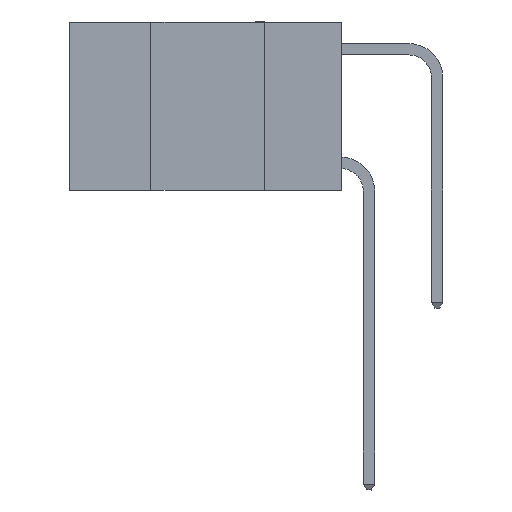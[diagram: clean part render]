
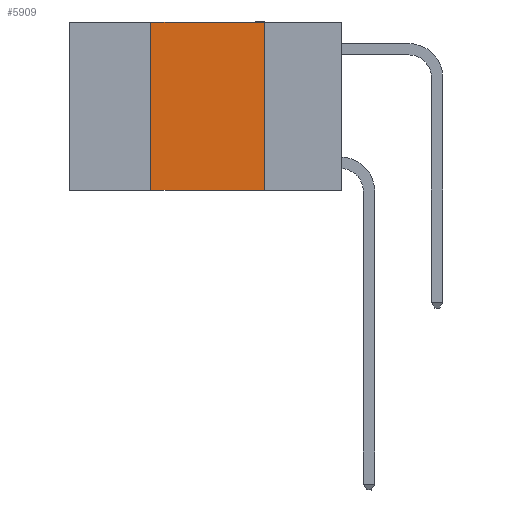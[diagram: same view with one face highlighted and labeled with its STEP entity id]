
A CAD part, left-side view. The second image highlights one B-rep face of the part: STEP entity #5909.
In plain terms, the highlighted planar face has unit normal (-1, 0, 0).
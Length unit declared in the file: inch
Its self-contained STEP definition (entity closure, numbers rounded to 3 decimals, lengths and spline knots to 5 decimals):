
#343 = VERTEX_POINT ( 'NONE', #6708 ) ;
#415 = VECTOR ( 'NONE', #12996, 39.37008 ) ;
#549 = CARTESIAN_POINT ( 'NONE',  ( 0., 0.17, 0. ) ) ;
#1062 = ORIENTED_EDGE ( 'NONE', *, *, #9405, .F. ) ;
#1508 = AXIS2_PLACEMENT_3D ( 'NONE', #9633, #1908, #12872 ) ;
#1541 = ORIENTED_EDGE ( 'NONE', *, *, #9447, .F. ) ;
#1908 = DIRECTION ( 'NONE',  ( 1., 0., 0. ) ) ;
#2090 = FACE_OUTER_BOUND ( 'NONE', #12946, .T. ) ;
#2152 = DIRECTION ( 'NONE',  ( 0., 0., 1. ) ) ;
#2415 = VECTOR ( 'NONE', #8835, 39.37008 ) ;
#2990 = VERTEX_POINT ( 'NONE', #5222 ) ;
#5222 = CARTESIAN_POINT ( 'NONE',  ( 0., 0.42, -0.37 ) ) ;
#5909 = ADVANCED_FACE ( 'NONE', ( #2090 ), #18929, .F. ) ;
#6468 = LINE ( 'NONE', #7260, #2415 ) ;
#6708 = CARTESIAN_POINT ( 'NONE',  ( 0., 0.17, 0. ) ) ;
#7260 = CARTESIAN_POINT ( 'NONE',  ( 0., 0.6, 0. ) ) ;
#7269 = CARTESIAN_POINT ( 'NONE',  ( 0., 0.17, -0.37 ) ) ;
#8835 = DIRECTION ( 'NONE',  ( 0., -1., 0. ) ) ;
#9405 = EDGE_CURVE ( 'NONE', #343, #10947, #12389, .T. ) ;
#9447 = EDGE_CURVE ( 'NONE', #2990, #9771, #11911, .T. ) ;
#9500 = EDGE_CURVE ( 'NONE', #2990, #10947, #18613, .T. ) ;
#9633 = CARTESIAN_POINT ( 'NONE',  ( 0., 0.6, 0. ) ) ;
#9771 = VERTEX_POINT ( 'NONE', #17113 ) ;
#9808 = ORIENTED_EDGE ( 'NONE', *, *, #9500, .T. ) ;
#10111 = DIRECTION ( 'NONE',  ( 0., -1., 0. ) ) ;
#10947 = VERTEX_POINT ( 'NONE', #7269 ) ;
#11392 = VECTOR ( 'NONE', #2152, 39.37008 ) ;
#11579 = CARTESIAN_POINT ( 'NONE',  ( 0., 0.42, 0. ) ) ;
#11911 = LINE ( 'NONE', #11579, #11392 ) ;
#12389 = LINE ( 'NONE', #549, #415 ) ;
#12872 = DIRECTION ( 'NONE',  ( 0., 0., -1. ) ) ;
#12946 = EDGE_LOOP ( 'NONE', ( #1062, #13564, #1541, #9808 ) ) ;
#12996 = DIRECTION ( 'NONE',  ( 0., 0., -1. ) ) ;
#13564 = ORIENTED_EDGE ( 'NONE', *, *, #16190, .F. ) ;
#14599 = VECTOR ( 'NONE', #10111, 39.37008 ) ;
#14822 = CARTESIAN_POINT ( 'NONE',  ( 0., 0.6, -0.37 ) ) ;
#16190 = EDGE_CURVE ( 'NONE', #9771, #343, #6468, .T. ) ;
#17113 = CARTESIAN_POINT ( 'NONE',  ( 0., 0.42, 0. ) ) ;
#18613 = LINE ( 'NONE', #14822, #14599 ) ;
#18929 = PLANE ( 'NONE',  #1508 ) ;
